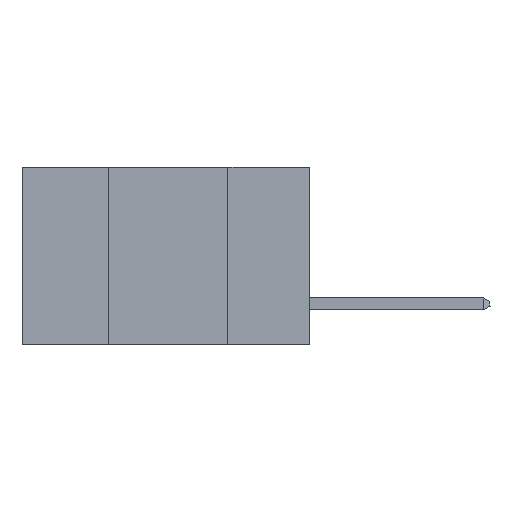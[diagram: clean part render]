
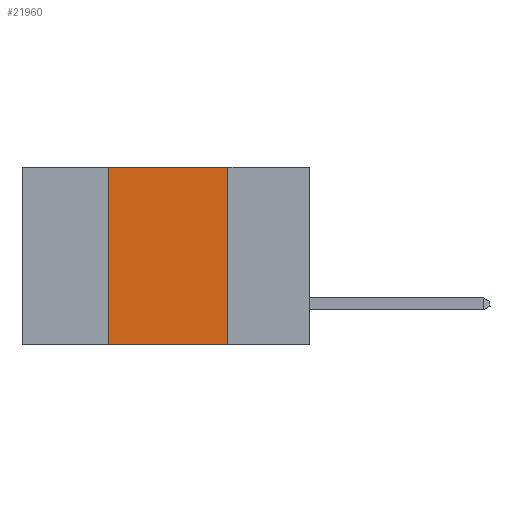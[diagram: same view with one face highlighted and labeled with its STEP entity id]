
A CAD part, left-side view. The second image highlights one B-rep face of the part: STEP entity #21960.
In plain terms, the highlighted planar face has unit normal (-1, 0, 0).
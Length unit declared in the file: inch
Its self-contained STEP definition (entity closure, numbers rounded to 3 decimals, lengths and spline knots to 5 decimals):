
#1136 = VECTOR ( 'NONE', #15367, 39.37008 ) ;
#1214 = CARTESIAN_POINT ( 'NONE',  ( 0., 0.42, 0. ) ) ;
#1240 = ORIENTED_EDGE ( 'NONE', *, *, #13104, .F. ) ;
#2005 = VERTEX_POINT ( 'NONE', #16400 ) ;
#2409 = EDGE_CURVE ( 'NONE', #2005, #20979, #5036, .T. ) ;
#2986 = DIRECTION ( 'NONE',  ( 0., 0., 1. ) ) ;
#3254 = ORIENTED_EDGE ( 'NONE', *, *, #2409, .F. ) ;
#3329 = EDGE_CURVE ( 'NONE', #13154, #20979, #11932, .T. ) ;
#4524 = ORIENTED_EDGE ( 'NONE', *, *, #6550, .F. ) ;
#4911 = AXIS2_PLACEMENT_3D ( 'NONE', #6477, #13390, #17245 ) ;
#5036 = LINE ( 'NONE', #6066, #1136 ) ;
#5087 = FACE_OUTER_BOUND ( 'NONE', #14894, .T. ) ;
#5544 = VECTOR ( 'NONE', #16892, 39.37008 ) ;
#6066 = CARTESIAN_POINT ( 'NONE',  ( 0., 0.17, 0. ) ) ;
#6400 = PLANE ( 'NONE',  #4911 ) ;
#6477 = CARTESIAN_POINT ( 'NONE',  ( 0., 0.6, 0. ) ) ;
#6550 = EDGE_CURVE ( 'NONE', #13154, #15713, #7640, .T. ) ;
#7640 = LINE ( 'NONE', #1214, #9837 ) ;
#9837 = VECTOR ( 'NONE', #2986, 39.37008 ) ;
#10888 = ORIENTED_EDGE ( 'NONE', *, *, #3329, .T. ) ;
#11560 = CARTESIAN_POINT ( 'NONE',  ( 0., 0.6, -0.37 ) ) ;
#11932 = LINE ( 'NONE', #11560, #5544 ) ;
#12392 = VECTOR ( 'NONE', #17858, 39.37008 ) ;
#13104 = EDGE_CURVE ( 'NONE', #15713, #2005, #14878, .T. ) ;
#13154 = VERTEX_POINT ( 'NONE', #14319 ) ;
#13390 = DIRECTION ( 'NONE',  ( 1., 0., 0. ) ) ;
#14319 = CARTESIAN_POINT ( 'NONE',  ( 0., 0.42, -0.37 ) ) ;
#14878 = LINE ( 'NONE', #21434, #12392 ) ;
#14894 = EDGE_LOOP ( 'NONE', ( #3254, #1240, #4524, #10888 ) ) ;
#15367 = DIRECTION ( 'NONE',  ( 0., 0., -1. ) ) ;
#15713 = VERTEX_POINT ( 'NONE', #22596 ) ;
#15884 = CARTESIAN_POINT ( 'NONE',  ( 0., 0.17, -0.37 ) ) ;
#16400 = CARTESIAN_POINT ( 'NONE',  ( 0., 0.17, 0. ) ) ;
#16892 = DIRECTION ( 'NONE',  ( 0., -1., 0. ) ) ;
#17245 = DIRECTION ( 'NONE',  ( 0., 0., -1. ) ) ;
#17858 = DIRECTION ( 'NONE',  ( 0., -1., 0. ) ) ;
#20979 = VERTEX_POINT ( 'NONE', #15884 ) ;
#21434 = CARTESIAN_POINT ( 'NONE',  ( 0., 0.6, 0. ) ) ;
#21960 = ADVANCED_FACE ( 'NONE', ( #5087 ), #6400, .F. ) ;
#22596 = CARTESIAN_POINT ( 'NONE',  ( 0., 0.42, 0. ) ) ;
